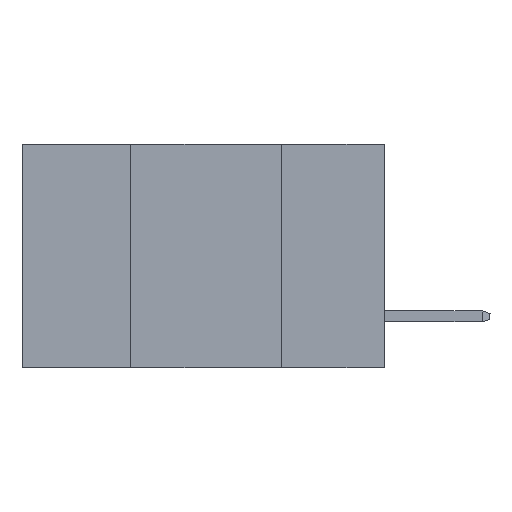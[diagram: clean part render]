
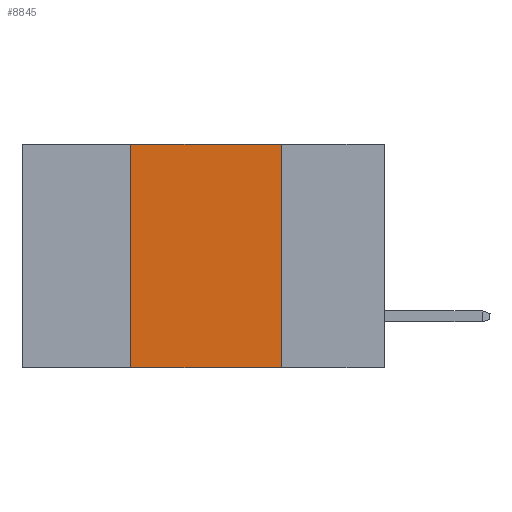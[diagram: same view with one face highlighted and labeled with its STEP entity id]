
A CAD part, left-side view. The second image highlights one B-rep face of the part: STEP entity #8845.
In plain terms, the highlighted planar face has unit normal (-1, 0, 0).
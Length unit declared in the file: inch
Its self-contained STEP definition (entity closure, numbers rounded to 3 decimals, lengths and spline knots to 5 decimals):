
#197 = VECTOR ( 'NONE', #5011, 39.37008 ) ;
#277 = CARTESIAN_POINT ( 'NONE',  ( 0., 0.6, 0. ) ) ;
#425 = ORIENTED_EDGE ( 'NONE', *, *, #5761, .F. ) ;
#622 = LINE ( 'NONE', #4134, #2468 ) ;
#628 = VERTEX_POINT ( 'NONE', #7858 ) ;
#787 = VECTOR ( 'NONE', #3738, 39.37008 ) ;
#874 = FACE_OUTER_BOUND ( 'NONE', #4206, .T. ) ;
#1186 = VERTEX_POINT ( 'NONE', #4315 ) ;
#1510 = DIRECTION ( 'NONE',  ( 0., 0., -1. ) ) ;
#1603 = EDGE_CURVE ( 'NONE', #628, #10865, #622, .T. ) ;
#1780 = VERTEX_POINT ( 'NONE', #4519 ) ;
#2085 = ORIENTED_EDGE ( 'NONE', *, *, #2223, .F. ) ;
#2223 = EDGE_CURVE ( 'NONE', #1186, #1780, #4903, .T. ) ;
#2468 = VECTOR ( 'NONE', #1510, 39.37008 ) ;
#3313 = PLANE ( 'NONE',  #9454 ) ;
#3738 = DIRECTION ( 'NONE',  ( 0., -1., 0. ) ) ;
#4134 = CARTESIAN_POINT ( 'NONE',  ( 0., 0.17, -0.37 ) ) ;
#4206 = EDGE_LOOP ( 'NONE', ( #4251, #425, #2085, #7761 ) ) ;
#4251 = ORIENTED_EDGE ( 'NONE', *, *, #1603, .F. ) ;
#4315 = CARTESIAN_POINT ( 'NONE',  ( 0., 0.42, -0.37 ) ) ;
#4519 = CARTESIAN_POINT ( 'NONE',  ( 0., 0.42, 0. ) ) ;
#4546 = LINE ( 'NONE', #277, #7736 ) ;
#4788 = LINE ( 'NONE', #10499, #787 ) ;
#4903 = LINE ( 'NONE', #6505, #197 ) ;
#5011 = DIRECTION ( 'NONE',  ( 0., 0., 1. ) ) ;
#5761 = EDGE_CURVE ( 'NONE', #1780, #628, #4546, .T. ) ;
#5922 = CARTESIAN_POINT ( 'NONE',  ( 0., 0.6, 0. ) ) ;
#6505 = CARTESIAN_POINT ( 'NONE',  ( 0., 0.42, -0.37 ) ) ;
#7736 = VECTOR ( 'NONE', #8695, 39.37008 ) ;
#7761 = ORIENTED_EDGE ( 'NONE', *, *, #9472, .T. ) ;
#7799 = DIRECTION ( 'NONE',  ( 1., 0., 0. ) ) ;
#7858 = CARTESIAN_POINT ( 'NONE',  ( 0., 0.17, 0. ) ) ;
#8355 = CARTESIAN_POINT ( 'NONE',  ( 0., 0.17, -0.37 ) ) ;
#8580 = DIRECTION ( 'NONE',  ( 0., 0., -1. ) ) ;
#8695 = DIRECTION ( 'NONE',  ( 0., -1., 0. ) ) ;
#8845 = ADVANCED_FACE ( 'NONE', ( #874 ), #3313, .F. ) ;
#9454 = AXIS2_PLACEMENT_3D ( 'NONE', #5922, #7799, #8580 ) ;
#9472 = EDGE_CURVE ( 'NONE', #1186, #10865, #4788, .T. ) ;
#10499 = CARTESIAN_POINT ( 'NONE',  ( 0., 0.6, -0.37 ) ) ;
#10865 = VERTEX_POINT ( 'NONE', #8355 ) ;
